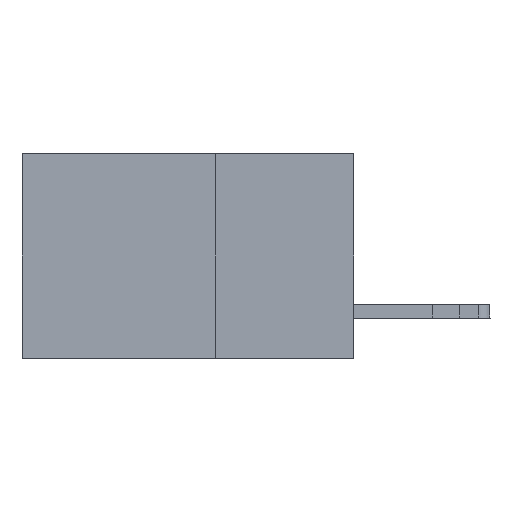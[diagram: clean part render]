
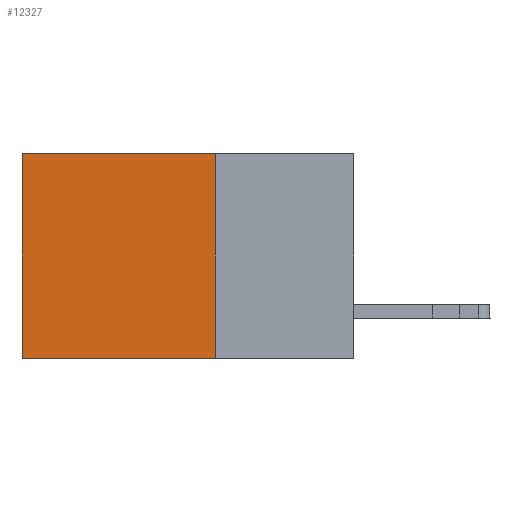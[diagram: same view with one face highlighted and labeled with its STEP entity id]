
A CAD part, left-side view. The second image highlights one B-rep face of the part: STEP entity #12327.
In plain terms, the highlighted planar face has unit normal (-1, 0, 0).
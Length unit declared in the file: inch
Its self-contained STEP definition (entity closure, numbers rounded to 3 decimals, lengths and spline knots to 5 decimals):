
#198 = EDGE_CURVE ( 'NONE', #13020, #1214, #8602, .T. ) ;
#243 = CARTESIAN_POINT ( 'NONE',  ( 0.2875, 0.6, -0.37 ) ) ;
#1214 = VERTEX_POINT ( 'NONE', #14396 ) ;
#1490 = DIRECTION ( 'NONE',  ( 0., 0., -1. ) ) ;
#2162 = EDGE_LOOP ( 'NONE', ( #23424, #21391, #12383, #11787 ) ) ;
#2196 = CARTESIAN_POINT ( 'NONE',  ( 0.2875, 0.25, -0.37 ) ) ;
#3124 = VECTOR ( 'NONE', #1490, 39.37008 ) ;
#3543 = EDGE_CURVE ( 'NONE', #23026, #13889, #4634, .T. ) ;
#4634 = LINE ( 'NONE', #12517, #10102 ) ;
#5440 = CARTESIAN_POINT ( 'NONE',  ( 0.2875, 0.25, 0. ) ) ;
#6398 = DIRECTION ( 'NONE',  ( 0., 1., 0. ) ) ;
#8410 = CARTESIAN_POINT ( 'NONE',  ( 0.2875, 0.25, 0. ) ) ;
#8602 = LINE ( 'NONE', #5440, #9551 ) ;
#8733 = DIRECTION ( 'NONE',  ( 0., 1., 0. ) ) ;
#9551 = VECTOR ( 'NONE', #8733, 39.37008 ) ;
#10102 = VECTOR ( 'NONE', #6398, 39.37008 ) ;
#10411 = PLANE ( 'NONE',  #10646 ) ;
#10646 = AXIS2_PLACEMENT_3D ( 'NONE', #8410, #12290, #12668 ) ;
#11774 = VECTOR ( 'NONE', #17418, 39.37008 ) ;
#11787 = ORIENTED_EDGE ( 'NONE', *, *, #198, .T. ) ;
#12290 = DIRECTION ( 'NONE',  ( 1., 0., 0. ) ) ;
#12327 = ADVANCED_FACE ( 'NONE', ( #19799 ), #10411, .F. ) ;
#12383 = ORIENTED_EDGE ( 'NONE', *, *, #14162, .F. ) ;
#12517 = CARTESIAN_POINT ( 'NONE',  ( 0.2875, 0.25, -0.37 ) ) ;
#12668 = DIRECTION ( 'NONE',  ( 0., 0., -1. ) ) ;
#13020 = VERTEX_POINT ( 'NONE', #19253 ) ;
#13661 = CARTESIAN_POINT ( 'NONE',  ( 0.2875, 0.6, 0. ) ) ;
#13889 = VERTEX_POINT ( 'NONE', #243 ) ;
#14162 = EDGE_CURVE ( 'NONE', #13020, #23026, #24644, .T. ) ;
#14396 = CARTESIAN_POINT ( 'NONE',  ( 0.2875, 0.6, 0. ) ) ;
#17418 = DIRECTION ( 'NONE',  ( 0., 0., -1. ) ) ;
#19253 = CARTESIAN_POINT ( 'NONE',  ( 0.2875, 0.25, 0. ) ) ;
#19799 = FACE_OUTER_BOUND ( 'NONE', #2162, .T. ) ;
#21391 = ORIENTED_EDGE ( 'NONE', *, *, #3543, .F. ) ;
#23026 = VERTEX_POINT ( 'NONE', #2196 ) ;
#23046 = LINE ( 'NONE', #13661, #11774 ) ;
#23424 = ORIENTED_EDGE ( 'NONE', *, *, #23818, .T. ) ;
#23818 = EDGE_CURVE ( 'NONE', #1214, #13889, #23046, .T. ) ;
#24403 = CARTESIAN_POINT ( 'NONE',  ( 0.2875, 0.25, 0. ) ) ;
#24644 = LINE ( 'NONE', #24403, #3124 ) ;
